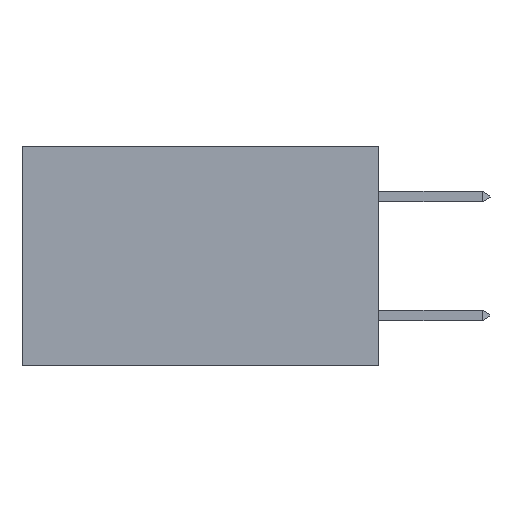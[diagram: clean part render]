
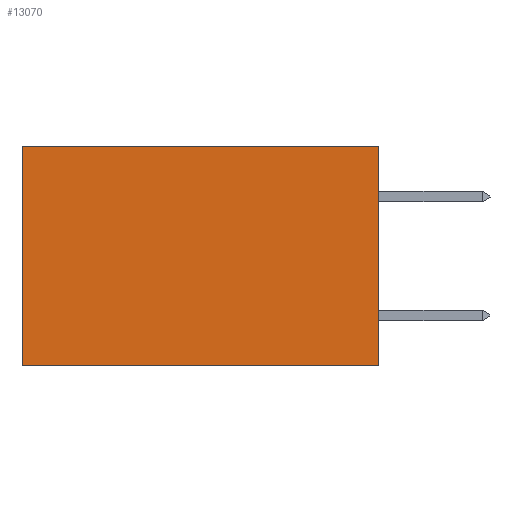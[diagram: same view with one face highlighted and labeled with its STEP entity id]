
A CAD part, left-side view. The second image highlights one B-rep face of the part: STEP entity #13070.
In plain terms, the highlighted planar face has unit normal (-1, 0, 0).
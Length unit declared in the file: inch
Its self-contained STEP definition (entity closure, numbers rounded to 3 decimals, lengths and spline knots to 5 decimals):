
#22 = VECTOR ( 'NONE', #26721, 39.37008 ) ;
#713 = PLANE ( 'NONE',  #2501 ) ;
#749 = LINE ( 'NONE', #15586, #22 ) ;
#2098 = CARTESIAN_POINT ( 'NONE',  ( 0.298, 0.6, 0. ) ) ;
#2306 = DIRECTION ( 'NONE',  ( 0., 0., -1. ) ) ;
#2501 = AXIS2_PLACEMENT_3D ( 'NONE', #16564, #3007, #18803 ) ;
#2849 = ORIENTED_EDGE ( 'NONE', *, *, #22757, .T. ) ;
#3007 = DIRECTION ( 'NONE',  ( 1., 0., 0. ) ) ;
#3798 = ORIENTED_EDGE ( 'NONE', *, *, #13352, .F. ) ;
#3962 = LINE ( 'NONE', #2098, #15301 ) ;
#4360 = DIRECTION ( 'NONE',  ( 0., 0., -1. ) ) ;
#6079 = DIRECTION ( 'NONE',  ( 0., 1., 0. ) ) ;
#6582 = CARTESIAN_POINT ( 'NONE',  ( 0.298, 0., -0.37 ) ) ;
#6769 = CARTESIAN_POINT ( 'NONE',  ( 0.298, 0., 0. ) ) ;
#7573 = EDGE_CURVE ( 'NONE', #25384, #25848, #749, .T. ) ;
#7819 = FACE_OUTER_BOUND ( 'NONE', #23844, .T. ) ;
#8742 = VERTEX_POINT ( 'NONE', #15029 ) ;
#9085 = CARTESIAN_POINT ( 'NONE',  ( 0.298, 0., 0. ) ) ;
#13070 = ADVANCED_FACE ( 'NONE', ( #7819 ), #713, .F. ) ;
#13352 = EDGE_CURVE ( 'NONE', #21044, #8742, #19419, .T. ) ;
#15029 = CARTESIAN_POINT ( 'NONE',  ( 0.298, 0.6, -0.37 ) ) ;
#15160 = CARTESIAN_POINT ( 'NONE',  ( 0.298, 0., -0.37 ) ) ;
#15301 = VECTOR ( 'NONE', #4360, 39.37008 ) ;
#15586 = CARTESIAN_POINT ( 'NONE',  ( 0.298, 0., 0. ) ) ;
#16564 = CARTESIAN_POINT ( 'NONE',  ( 0.298, 0., 0. ) ) ;
#18032 = VECTOR ( 'NONE', #6079, 39.37008 ) ;
#18803 = DIRECTION ( 'NONE',  ( 0., 0., -1. ) ) ;
#18886 = VECTOR ( 'NONE', #2306, 39.37008 ) ;
#19419 = LINE ( 'NONE', #15160, #18032 ) ;
#19578 = CARTESIAN_POINT ( 'NONE',  ( 0.298, 0.6, 0. ) ) ;
#21044 = VERTEX_POINT ( 'NONE', #6582 ) ;
#22757 = EDGE_CURVE ( 'NONE', #25848, #8742, #3962, .T. ) ;
#23028 = ORIENTED_EDGE ( 'NONE', *, *, #26086, .F. ) ;
#23714 = ORIENTED_EDGE ( 'NONE', *, *, #7573, .T. ) ;
#23844 = EDGE_LOOP ( 'NONE', ( #2849, #3798, #23028, #23714 ) ) ;
#24821 = LINE ( 'NONE', #6769, #18886 ) ;
#25384 = VERTEX_POINT ( 'NONE', #9085 ) ;
#25848 = VERTEX_POINT ( 'NONE', #19578 ) ;
#26086 = EDGE_CURVE ( 'NONE', #25384, #21044, #24821, .T. ) ;
#26721 = DIRECTION ( 'NONE',  ( 0., 1., 0. ) ) ;
